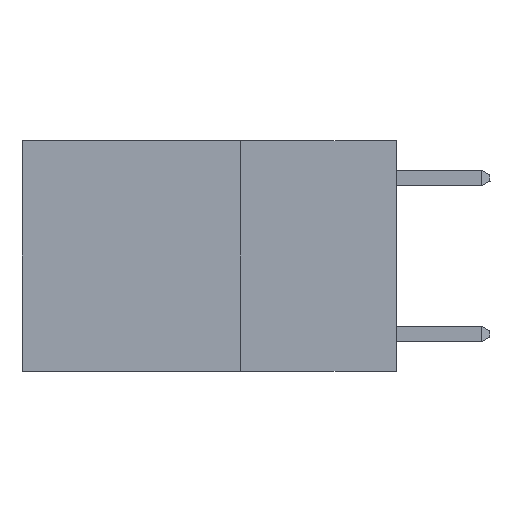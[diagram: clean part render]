
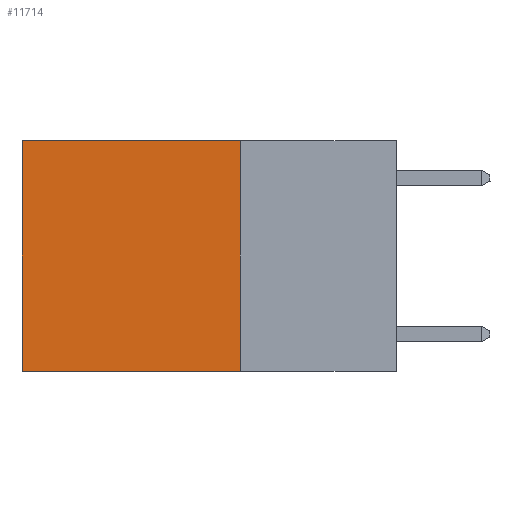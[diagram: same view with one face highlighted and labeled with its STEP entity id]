
A CAD part, left-side view. The second image highlights one B-rep face of the part: STEP entity #11714.
In plain terms, the highlighted planar face has unit normal (-1, 0, 0).
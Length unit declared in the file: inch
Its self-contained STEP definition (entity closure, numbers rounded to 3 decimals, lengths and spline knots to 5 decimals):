
#171 = DIRECTION ( 'NONE',  ( 0., 0., -1. ) ) ;
#643 = VERTEX_POINT ( 'NONE', #12611 ) ;
#1777 = VECTOR ( 'NONE', #18139, 39.37008 ) ;
#2250 = ORIENTED_EDGE ( 'NONE', *, *, #8033, .T. ) ;
#2477 = LINE ( 'NONE', #11300, #1777 ) ;
#2596 = EDGE_CURVE ( 'NONE', #18859, #643, #14568, .T. ) ;
#4018 = VERTEX_POINT ( 'NONE', #10289 ) ;
#5061 = DIRECTION ( 'NONE',  ( 0., 1., 0. ) ) ;
#5477 = EDGE_CURVE ( 'NONE', #4018, #8491, #2477, .T. ) ;
#6519 = VECTOR ( 'NONE', #5061, 39.37008 ) ;
#8033 = EDGE_CURVE ( 'NONE', #4018, #18859, #13098, .T. ) ;
#8196 = FACE_OUTER_BOUND ( 'NONE', #27302, .T. ) ;
#8491 = VERTEX_POINT ( 'NONE', #17502 ) ;
#10099 = AXIS2_PLACEMENT_3D ( 'NONE', #19026, #19602, #12707 ) ;
#10289 = CARTESIAN_POINT ( 'NONE',  ( 0.2625, 0.25, 0. ) ) ;
#11300 = CARTESIAN_POINT ( 'NONE',  ( 0.2625, 0.25, 0. ) ) ;
#11714 = ADVANCED_FACE ( 'NONE', ( #8196 ), #25569, .F. ) ;
#12611 = CARTESIAN_POINT ( 'NONE',  ( 0.2625, 0.6, -0.37 ) ) ;
#12707 = DIRECTION ( 'NONE',  ( 0., 0., -1. ) ) ;
#12715 = CARTESIAN_POINT ( 'NONE',  ( 0.2625, 0.25, 0. ) ) ;
#13098 = LINE ( 'NONE', #12715, #18981 ) ;
#13132 = DIRECTION ( 'NONE',  ( 0., 1., 0. ) ) ;
#13451 = CARTESIAN_POINT ( 'NONE',  ( 0.2625, 0.6, 0. ) ) ;
#14568 = LINE ( 'NONE', #13451, #17297 ) ;
#15152 = ORIENTED_EDGE ( 'NONE', *, *, #5477, .F. ) ;
#15423 = CARTESIAN_POINT ( 'NONE',  ( 0.2625, 0.6, 0. ) ) ;
#16554 = LINE ( 'NONE', #24849, #6519 ) ;
#17297 = VECTOR ( 'NONE', #171, 39.37008 ) ;
#17502 = CARTESIAN_POINT ( 'NONE',  ( 0.2625, 0.25, -0.37 ) ) ;
#18046 = ORIENTED_EDGE ( 'NONE', *, *, #26708, .F. ) ;
#18139 = DIRECTION ( 'NONE',  ( 0., 0., -1. ) ) ;
#18859 = VERTEX_POINT ( 'NONE', #15423 ) ;
#18981 = VECTOR ( 'NONE', #13132, 39.37008 ) ;
#19026 = CARTESIAN_POINT ( 'NONE',  ( 0.2625, 0.25, 0. ) ) ;
#19602 = DIRECTION ( 'NONE',  ( 1., 0., 0. ) ) ;
#21742 = ORIENTED_EDGE ( 'NONE', *, *, #2596, .T. ) ;
#24849 = CARTESIAN_POINT ( 'NONE',  ( 0.2625, 0.25, -0.37 ) ) ;
#25569 = PLANE ( 'NONE',  #10099 ) ;
#26708 = EDGE_CURVE ( 'NONE', #8491, #643, #16554, .T. ) ;
#27302 = EDGE_LOOP ( 'NONE', ( #21742, #18046, #15152, #2250 ) ) ;
